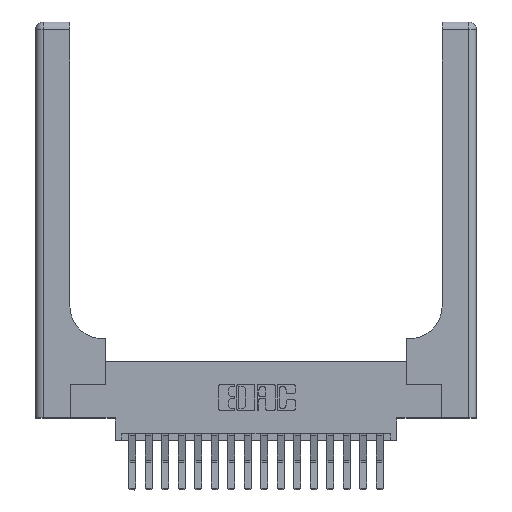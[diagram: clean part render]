
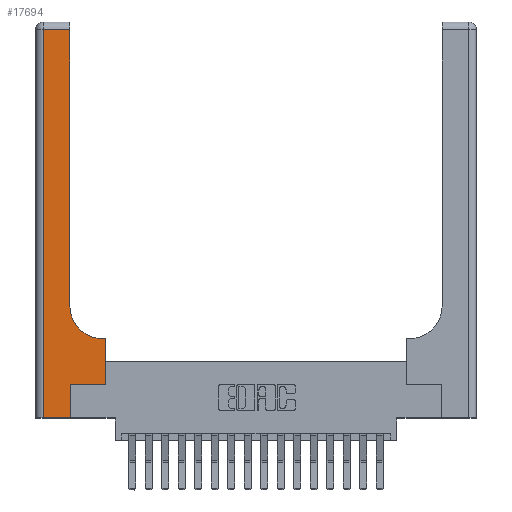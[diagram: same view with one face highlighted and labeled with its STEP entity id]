
A CAD part, top view. The second image highlights one B-rep face of the part: STEP entity #17694.
In plain terms, the highlighted planar face has unit normal (0, 0, 1).
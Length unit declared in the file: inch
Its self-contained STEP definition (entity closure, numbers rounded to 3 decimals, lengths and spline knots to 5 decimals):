
#65 = CIRCLE ( 'NONE', #12700, 0.25 ) ;
#192 = CARTESIAN_POINT ( 'NONE',  ( 0.06, 3., 0.37 ) ) ;
#346 = DIRECTION ( 'NONE',  ( 1., 0., 0. ) ) ;
#452 = DIRECTION ( 'NONE',  ( 0., -1., 0. ) ) ;
#586 = CARTESIAN_POINT ( 'NONE',  ( 0.26, 0.6, 0.37 ) ) ;
#1181 = CARTESIAN_POINT ( 'NONE',  ( 0., 2.94, 0.37 ) ) ;
#1240 = EDGE_CURVE ( 'NONE', #1890, #1639, #65, .T. ) ;
#1322 = CARTESIAN_POINT ( 'NONE',  ( 0.26, 0.85, 0.37 ) ) ;
#1639 = VERTEX_POINT ( 'NONE', #1322 ) ;
#1733 = EDGE_CURVE ( 'NONE', #4595, #7793, #8068, .T. ) ;
#1890 = VERTEX_POINT ( 'NONE', #6758 ) ;
#1893 = LINE ( 'NONE', #1181, #15633 ) ;
#1963 = LINE ( 'NONE', #5531, #9961 ) ;
#2092 = VERTEX_POINT ( 'NONE', #13209 ) ;
#2413 = EDGE_CURVE ( 'NONE', #3252, #8041, #17139, .T. ) ;
#2547 = EDGE_CURVE ( 'NONE', #4923, #3252, #3814, .T. ) ;
#2559 = DIRECTION ( 'NONE',  ( 0., 1., 0. ) ) ;
#2694 = DIRECTION ( 'NONE',  ( -1., 0., 0. ) ) ;
#3123 = VECTOR ( 'NONE', #5291, 39.37008 ) ;
#3252 = VERTEX_POINT ( 'NONE', #9911 ) ;
#3389 = CARTESIAN_POINT ( 'NONE',  ( 0., 0., 0.37 ) ) ;
#3814 = LINE ( 'NONE', #15655, #3123 ) ;
#3868 = ORIENTED_EDGE ( 'NONE', *, *, #2547, .T. ) ;
#3946 = CARTESIAN_POINT ( 'NONE',  ( 0.26, 2.94, 0.37 ) ) ;
#4216 = EDGE_CURVE ( 'NONE', #7793, #4923, #4938, .T. ) ;
#4595 = VERTEX_POINT ( 'NONE', #5199 ) ;
#4923 = VERTEX_POINT ( 'NONE', #15046 ) ;
#4938 = LINE ( 'NONE', #3389, #12877 ) ;
#4939 = CARTESIAN_POINT ( 'NONE',  ( 0.528, 0.25, 0.37 ) ) ;
#5199 = CARTESIAN_POINT ( 'NONE',  ( 0.06, 2.94, 0.37 ) ) ;
#5203 = FACE_OUTER_BOUND ( 'NONE', #11804, .T. ) ;
#5291 = DIRECTION ( 'NONE',  ( 0., 1., 0. ) ) ;
#5531 = CARTESIAN_POINT ( 'NONE',  ( 0.528, 0.25, 0.37 ) ) ;
#5702 = VECTOR ( 'NONE', #6539, 39.37008 ) ;
#6318 = VERTEX_POINT ( 'NONE', #3946 ) ;
#6516 = DIRECTION ( 'NONE',  ( 1., 0., 0. ) ) ;
#6536 = DIRECTION ( 'NONE',  ( 0., 0., -1. ) ) ;
#6539 = DIRECTION ( 'NONE',  ( 1., 0., 0. ) ) ;
#6552 = CARTESIAN_POINT ( 'NONE',  ( 0.51, 0.85, 0.37 ) ) ;
#6592 = DIRECTION ( 'NONE',  ( -1., 0., 0. ) ) ;
#6758 = CARTESIAN_POINT ( 'NONE',  ( 0.51, 0.6, 0.37 ) ) ;
#7730 = AXIS2_PLACEMENT_3D ( 'NONE', #8060, #18472, #9564 ) ;
#7793 = VERTEX_POINT ( 'NONE', #11948 ) ;
#8041 = VERTEX_POINT ( 'NONE', #4939 ) ;
#8060 = CARTESIAN_POINT ( 'NONE',  ( 0., 3., 0.37 ) ) ;
#8068 = LINE ( 'NONE', #192, #18996 ) ;
#8499 = ORIENTED_EDGE ( 'NONE', *, *, #4216, .T. ) ;
#8511 = ORIENTED_EDGE ( 'NONE', *, *, #1733, .T. ) ;
#8674 = VECTOR ( 'NONE', #6592, 39.37008 ) ;
#8753 = LINE ( 'NONE', #12978, #11806 ) ;
#9564 = DIRECTION ( 'NONE',  ( -1., 0., 0. ) ) ;
#9911 = CARTESIAN_POINT ( 'NONE',  ( 0.265, 0.25, 0.37 ) ) ;
#9961 = VECTOR ( 'NONE', #14463, 39.37008 ) ;
#10226 = ORIENTED_EDGE ( 'NONE', *, *, #15889, .T. ) ;
#11804 = EDGE_LOOP ( 'NONE', ( #18883, #17569, #8511, #8499, #3868, #13834, #10226, #15843, #13877 ) ) ;
#11806 = VECTOR ( 'NONE', #2559, 39.37008 ) ;
#11948 = CARTESIAN_POINT ( 'NONE',  ( 0.06, 0., 0.37 ) ) ;
#12514 = PLANE ( 'NONE',  #7730 ) ;
#12669 = EDGE_CURVE ( 'NONE', #2092, #1890, #16604, .T. ) ;
#12700 = AXIS2_PLACEMENT_3D ( 'NONE', #6552, #6536, #6516 ) ;
#12877 = VECTOR ( 'NONE', #346, 39.37008 ) ;
#12978 = CARTESIAN_POINT ( 'NONE',  ( 0.26, 3., 0.37 ) ) ;
#13209 = CARTESIAN_POINT ( 'NONE',  ( 0.528, 0.6, 0.37 ) ) ;
#13834 = ORIENTED_EDGE ( 'NONE', *, *, #2413, .T. ) ;
#13877 = ORIENTED_EDGE ( 'NONE', *, *, #1240, .T. ) ;
#14463 = DIRECTION ( 'NONE',  ( 0., 1., 0. ) ) ;
#15046 = CARTESIAN_POINT ( 'NONE',  ( 0.265, 0., 0.37 ) ) ;
#15469 = CARTESIAN_POINT ( 'NONE',  ( 0.265, 0.25, 0.37 ) ) ;
#15633 = VECTOR ( 'NONE', #2694, 39.37008 ) ;
#15655 = CARTESIAN_POINT ( 'NONE',  ( 0.265, 0., 0.37 ) ) ;
#15843 = ORIENTED_EDGE ( 'NONE', *, *, #12669, .T. ) ;
#15889 = EDGE_CURVE ( 'NONE', #8041, #2092, #1963, .T. ) ;
#16604 = LINE ( 'NONE', #586, #8674 ) ;
#16755 = EDGE_CURVE ( 'NONE', #1639, #6318, #8753, .T. ) ;
#17139 = LINE ( 'NONE', #15469, #5702 ) ;
#17569 = ORIENTED_EDGE ( 'NONE', *, *, #18615, .T. ) ;
#17694 = ADVANCED_FACE ( 'NONE', ( #5203 ), #12514, .F. ) ;
#18472 = DIRECTION ( 'NONE',  ( 0., 0., -1. ) ) ;
#18615 = EDGE_CURVE ( 'NONE', #6318, #4595, #1893, .T. ) ;
#18883 = ORIENTED_EDGE ( 'NONE', *, *, #16755, .T. ) ;
#18996 = VECTOR ( 'NONE', #452, 39.37008 ) ;
